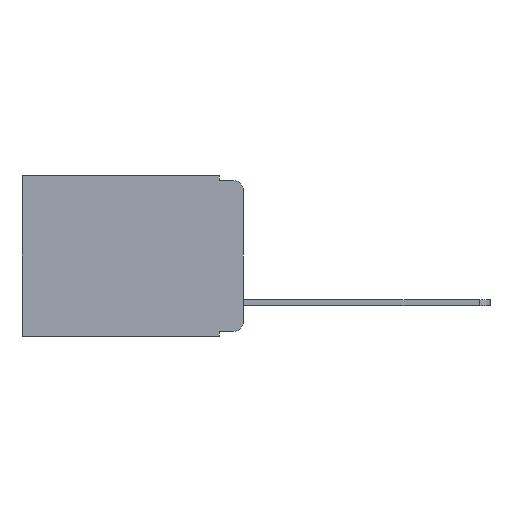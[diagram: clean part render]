
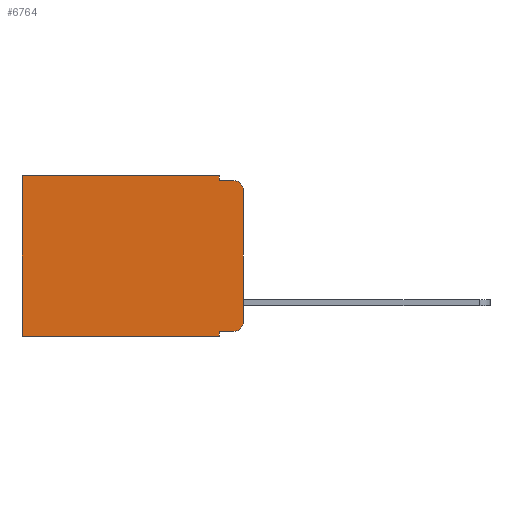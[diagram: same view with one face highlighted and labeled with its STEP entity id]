
A CAD part, left-side view. The second image highlights one B-rep face of the part: STEP entity #6764.
In plain terms, the highlighted planar face has unit normal (-1, 0, 0).
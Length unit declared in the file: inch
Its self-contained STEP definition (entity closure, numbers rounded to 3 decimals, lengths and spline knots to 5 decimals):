
#90 = VERTEX_POINT ( 'NONE', #481 ) ;
#238 = VECTOR ( 'NONE', #6954, 39.37008 ) ;
#254 = EDGE_CURVE ( 'NONE', #9399, #9348, #2015, .T. ) ;
#274 = EDGE_CURVE ( 'NONE', #9399, #6614, #8516, .T. ) ;
#481 = CARTESIAN_POINT ( 'NONE',  ( 0.298, 0., -0.03 ) ) ;
#521 = VECTOR ( 'NONE', #10566, 39.37008 ) ;
#630 = VECTOR ( 'NONE', #2219, 39.37008 ) ;
#919 = EDGE_CURVE ( 'NONE', #6614, #9951, #2712, .T. ) ;
#921 = AXIS2_PLACEMENT_3D ( 'NONE', #8666, #8735, #9699 ) ;
#929 = LINE ( 'NONE', #6464, #9702 ) ;
#956 = VERTEX_POINT ( 'NONE', #8354 ) ;
#1258 = EDGE_CURVE ( 'NONE', #90, #9951, #8496, .T. ) ;
#1441 = CARTESIAN_POINT ( 'NONE',  ( 0.298, 0.02, -0.333 ) ) ;
#1552 = CARTESIAN_POINT ( 'NONE',  ( 0.298, 0.051, 0. ) ) ;
#1817 = EDGE_CURVE ( 'NONE', #90, #956, #5656, .T. ) ;
#2015 = LINE ( 'NONE', #10115, #4628 ) ;
#2151 = EDGE_CURVE ( 'NONE', #9348, #8817, #5009, .T. ) ;
#2219 = DIRECTION ( 'NONE',  ( 0., 0., -1. ) ) ;
#2584 = ORIENTED_EDGE ( 'NONE', *, *, #1817, .F. ) ;
#2712 = LINE ( 'NONE', #10949, #238 ) ;
#2743 = VERTEX_POINT ( 'NONE', #1441 ) ;
#2858 = EDGE_CURVE ( 'NONE', #3063, #8817, #9716, .T. ) ;
#3063 = VERTEX_POINT ( 'NONE', #10170 ) ;
#3070 = DIRECTION ( 'NONE',  ( 0., 0., -1. ) ) ;
#3246 = PLANE ( 'NONE',  #6347 ) ;
#3289 = CARTESIAN_POINT ( 'NONE',  ( 0.298, 0.473, 0. ) ) ;
#3356 = EDGE_CURVE ( 'NONE', #7106, #3063, #3618, .T. ) ;
#3404 = VECTOR ( 'NONE', #9180, 39.37008 ) ;
#3423 = CARTESIAN_POINT ( 'NONE',  ( 0.298, 0.473, -0.343 ) ) ;
#3618 = LINE ( 'NONE', #5518, #630 ) ;
#3672 = ORIENTED_EDGE ( 'NONE', *, *, #254, .T. ) ;
#4099 = DIRECTION ( 'NONE',  ( 1., 0., 0. ) ) ;
#4156 = ORIENTED_EDGE ( 'NONE', *, *, #6190, .T. ) ;
#4316 = CARTESIAN_POINT ( 'NONE',  ( 0.298, 0.473, 0. ) ) ;
#4479 = ORIENTED_EDGE ( 'NONE', *, *, #4508, .T. ) ;
#4499 = DIRECTION ( 'NONE',  ( 0., 1., 0. ) ) ;
#4508 = EDGE_CURVE ( 'NONE', #7106, #2743, #929, .T. ) ;
#4628 = VECTOR ( 'NONE', #4988, 39.37008 ) ;
#4742 = CARTESIAN_POINT ( 'NONE',  ( 0.298, 0.051, -0.01 ) ) ;
#4988 = DIRECTION ( 'NONE',  ( 0., 1., 0. ) ) ;
#5009 = LINE ( 'NONE', #4316, #521 ) ;
#5148 = CARTESIAN_POINT ( 'NONE',  ( 0.298, 0.051, 0. ) ) ;
#5155 = ORIENTED_EDGE ( 'NONE', *, *, #1258, .T. ) ;
#5518 = CARTESIAN_POINT ( 'NONE',  ( 0.298, 0.051, 0. ) ) ;
#5656 = LINE ( 'NONE', #9581, #3404 ) ;
#5661 = ORIENTED_EDGE ( 'NONE', *, *, #274, .F. ) ;
#5823 = CARTESIAN_POINT ( 'NONE',  ( 0.298, 0.02, -0.01 ) ) ;
#5921 = ORIENTED_EDGE ( 'NONE', *, *, #2151, .T. ) ;
#6185 = ORIENTED_EDGE ( 'NONE', *, *, #2858, .F. ) ;
#6190 = EDGE_CURVE ( 'NONE', #2743, #956, #9660, .T. ) ;
#6337 = VECTOR ( 'NONE', #8046, 39.37008 ) ;
#6347 = AXIS2_PLACEMENT_3D ( 'NONE', #9066, #4099, #9874 ) ;
#6464 = CARTESIAN_POINT ( 'NONE',  ( 0.298, 0.051, -0.333 ) ) ;
#6614 = VERTEX_POINT ( 'NONE', #4742 ) ;
#6764 = ADVANCED_FACE ( 'NONE', ( #8886 ), #3246, .F. ) ;
#6954 = DIRECTION ( 'NONE',  ( 0., -1., 0. ) ) ;
#7063 = CARTESIAN_POINT ( 'NONE',  ( 0.298, 0.051, -0.333 ) ) ;
#7106 = VERTEX_POINT ( 'NONE', #7063 ) ;
#7603 = VECTOR ( 'NONE', #4499, 39.37008 ) ;
#7853 = CARTESIAN_POINT ( 'NONE',  ( 0.298, 0.02, -0.03 ) ) ;
#8046 = DIRECTION ( 'NONE',  ( 0., 0., -1. ) ) ;
#8354 = CARTESIAN_POINT ( 'NONE',  ( 0.298, 0., -0.313 ) ) ;
#8380 = ORIENTED_EDGE ( 'NONE', *, *, #3356, .F. ) ;
#8496 = CIRCLE ( 'NONE', #8965, 0.02 ) ;
#8516 = LINE ( 'NONE', #5148, #6337 ) ;
#8666 = CARTESIAN_POINT ( 'NONE',  ( 0.298, 0.02, -0.313 ) ) ;
#8735 = DIRECTION ( 'NONE',  ( -1., 0., 0. ) ) ;
#8766 = CARTESIAN_POINT ( 'NONE',  ( 0.298, 0., -0.343 ) ) ;
#8817 = VERTEX_POINT ( 'NONE', #3423 ) ;
#8886 = FACE_OUTER_BOUND ( 'NONE', #10802, .T. ) ;
#8908 = DIRECTION ( 'NONE',  ( -1., 0., 0. ) ) ;
#8965 = AXIS2_PLACEMENT_3D ( 'NONE', #7853, #8908, #3070 ) ;
#9066 = CARTESIAN_POINT ( 'NONE',  ( 0.298, 0., 0. ) ) ;
#9134 = DIRECTION ( 'NONE',  ( 0., -1., 0. ) ) ;
#9180 = DIRECTION ( 'NONE',  ( 0., 0., -1. ) ) ;
#9348 = VERTEX_POINT ( 'NONE', #3289 ) ;
#9399 = VERTEX_POINT ( 'NONE', #1552 ) ;
#9508 = ORIENTED_EDGE ( 'NONE', *, *, #919, .F. ) ;
#9581 = CARTESIAN_POINT ( 'NONE',  ( 0.298, 0., 0. ) ) ;
#9660 = CIRCLE ( 'NONE', #921, 0.02 ) ;
#9699 = DIRECTION ( 'NONE',  ( 0., 0., -1. ) ) ;
#9702 = VECTOR ( 'NONE', #9134, 39.37008 ) ;
#9716 = LINE ( 'NONE', #8766, #7603 ) ;
#9874 = DIRECTION ( 'NONE',  ( 0., 0., -1. ) ) ;
#9951 = VERTEX_POINT ( 'NONE', #5823 ) ;
#10115 = CARTESIAN_POINT ( 'NONE',  ( 0.298, 0., 0. ) ) ;
#10170 = CARTESIAN_POINT ( 'NONE',  ( 0.298, 0.051, -0.343 ) ) ;
#10566 = DIRECTION ( 'NONE',  ( 0., 0., -1. ) ) ;
#10802 = EDGE_LOOP ( 'NONE', ( #2584, #5155, #9508, #5661, #3672, #5921, #6185, #8380, #4479, #4156 ) ) ;
#10949 = CARTESIAN_POINT ( 'NONE',  ( 0.298, 0.051, -0.01 ) ) ;
